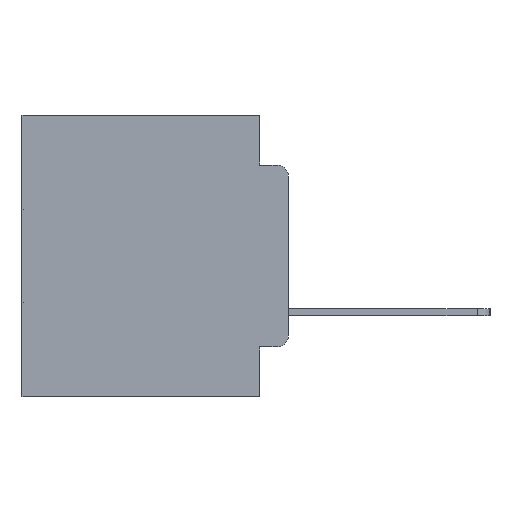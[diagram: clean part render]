
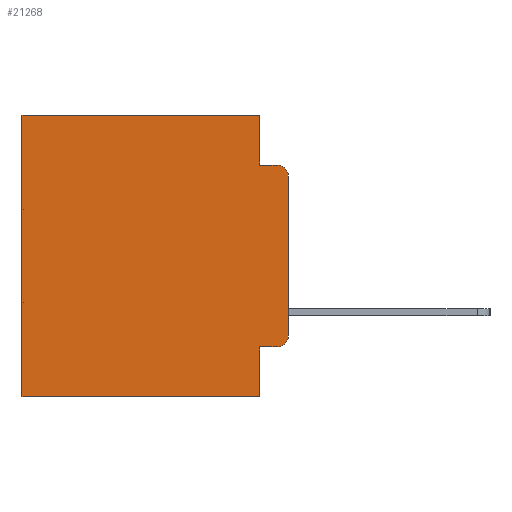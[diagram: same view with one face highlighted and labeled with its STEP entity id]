
A CAD part, left-side view. The second image highlights one B-rep face of the part: STEP entity #21268.
In plain terms, the highlighted planar face has unit normal (-1, 0, 0).
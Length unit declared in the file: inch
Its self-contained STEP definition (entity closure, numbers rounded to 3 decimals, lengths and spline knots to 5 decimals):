
#149 = VECTOR ( 'NONE', #6387, 39.37008 ) ;
#411 = ORIENTED_EDGE ( 'NONE', *, *, #12343, .F. ) ;
#608 = DIRECTION ( 'NONE',  ( 0., 0., -1. ) ) ;
#879 = DIRECTION ( 'NONE',  ( -1., 0., 0. ) ) ;
#1126 = AXIS2_PLACEMENT_3D ( 'NONE', #17650, #3889, #19891 ) ;
#2723 = VERTEX_POINT ( 'NONE', #9617 ) ;
#2884 = VECTOR ( 'NONE', #13279, 39.37008 ) ;
#2995 = ORIENTED_EDGE ( 'NONE', *, *, #27197, .T. ) ;
#3358 = EDGE_CURVE ( 'NONE', #24466, #16225, #23388, .T. ) ;
#3889 = DIRECTION ( 'NONE',  ( -1., 0., 0. ) ) ;
#4315 = VECTOR ( 'NONE', #608, 39.37008 ) ;
#4321 = EDGE_CURVE ( 'NONE', #2723, #8296, #20871, .T. ) ;
#4441 = ORIENTED_EDGE ( 'NONE', *, *, #24781, .F. ) ;
#5885 = ORIENTED_EDGE ( 'NONE', *, *, #16592, .T. ) ;
#5992 = LINE ( 'NONE', #10211, #21342 ) ;
#6387 = DIRECTION ( 'NONE',  ( 0., -1., 0. ) ) ;
#6478 = CARTESIAN_POINT ( 'NONE',  ( 0.298, 0.473, 0. ) ) ;
#6500 = VERTEX_POINT ( 'NONE', #8857 ) ;
#6699 = CARTESIAN_POINT ( 'NONE',  ( 0.298, 0., 0. ) ) ;
#7358 = VERTEX_POINT ( 'NONE', #14186 ) ;
#7810 = AXIS2_PLACEMENT_3D ( 'NONE', #22222, #10803, #13249 ) ;
#8296 = VERTEX_POINT ( 'NONE', #20118 ) ;
#8422 = VERTEX_POINT ( 'NONE', #9274 ) ;
#8857 = CARTESIAN_POINT ( 'NONE',  ( 0.298, 0.051, -0.4115 ) ) ;
#8985 = CARTESIAN_POINT ( 'NONE',  ( 0.298, 0., -0.1085 ) ) ;
#9028 = LINE ( 'NONE', #24500, #2884 ) ;
#9274 = CARTESIAN_POINT ( 'NONE',  ( 0.298, 0.051, -0.5 ) ) ;
#9549 = EDGE_CURVE ( 'NONE', #6500, #24466, #19239, .T. ) ;
#9617 = CARTESIAN_POINT ( 'NONE',  ( 0.298, 0.051, -0.0885 ) ) ;
#9822 = CARTESIAN_POINT ( 'NONE',  ( 0.298, 0.051, 0. ) ) ;
#9849 = ORIENTED_EDGE ( 'NONE', *, *, #4321, .F. ) ;
#10211 = CARTESIAN_POINT ( 'NONE',  ( 0.298, 0., 0. ) ) ;
#10475 = LINE ( 'NONE', #9822, #4315 ) ;
#10803 = DIRECTION ( 'NONE',  ( 1., 0., 0. ) ) ;
#10911 = PLANE ( 'NONE',  #7810 ) ;
#11896 = LINE ( 'NONE', #19379, #17164 ) ;
#12021 = CARTESIAN_POINT ( 'NONE',  ( 0.298, 0.473, 0. ) ) ;
#12343 = EDGE_CURVE ( 'NONE', #8422, #7358, #9028, .T. ) ;
#13090 = VERTEX_POINT ( 'NONE', #6478 ) ;
#13249 = DIRECTION ( 'NONE',  ( 0., 0., -1. ) ) ;
#13279 = DIRECTION ( 'NONE',  ( 0., 1., 0. ) ) ;
#13618 = DIRECTION ( 'NONE',  ( 0., -1., 0. ) ) ;
#14186 = CARTESIAN_POINT ( 'NONE',  ( 0.298, 0.473, -0.5 ) ) ;
#14570 = ORIENTED_EDGE ( 'NONE', *, *, #16103, .F. ) ;
#14743 = CARTESIAN_POINT ( 'NONE',  ( 0.298, 0.02, -0.3915 ) ) ;
#14925 = VECTOR ( 'NONE', #13618, 39.37008 ) ;
#15715 = EDGE_CURVE ( 'NONE', #6500, #8422, #11896, .T. ) ;
#16103 = EDGE_CURVE ( 'NONE', #23313, #16225, #16105, .T. ) ;
#16105 = LINE ( 'NONE', #6699, #20649 ) ;
#16225 = VERTEX_POINT ( 'NONE', #20453 ) ;
#16592 = EDGE_CURVE ( 'NONE', #26869, #13090, #5992, .T. ) ;
#16981 = DIRECTION ( 'NONE',  ( 0., 0., -1. ) ) ;
#17123 = DIRECTION ( 'NONE',  ( 0., 0., -1. ) ) ;
#17164 = VECTOR ( 'NONE', #17123, 39.37008 ) ;
#17650 = CARTESIAN_POINT ( 'NONE',  ( 0.298, 0.02, -0.1085 ) ) ;
#18629 = AXIS2_PLACEMENT_3D ( 'NONE', #14743, #879, #16981 ) ;
#18832 = FACE_OUTER_BOUND ( 'NONE', #26794, .T. ) ;
#19239 = LINE ( 'NONE', #20051, #149 ) ;
#19260 = DIRECTION ( 'NONE',  ( 0., 1., 0. ) ) ;
#19379 = CARTESIAN_POINT ( 'NONE',  ( 0.298, 0.051, 0. ) ) ;
#19891 = DIRECTION ( 'NONE',  ( 0., 0., -1. ) ) ;
#20051 = CARTESIAN_POINT ( 'NONE',  ( 0.298, 0.051, -0.4115 ) ) ;
#20118 = CARTESIAN_POINT ( 'NONE',  ( 0.298, 0.02, -0.0885 ) ) ;
#20185 = ORIENTED_EDGE ( 'NONE', *, *, #15715, .F. ) ;
#20218 = EDGE_CURVE ( 'NONE', #13090, #7358, #22135, .T. ) ;
#20269 = CARTESIAN_POINT ( 'NONE',  ( 0.298, 0.051, -0.0885 ) ) ;
#20453 = CARTESIAN_POINT ( 'NONE',  ( 0.298, 0., -0.3915 ) ) ;
#20495 = CARTESIAN_POINT ( 'NONE',  ( 0.298, 0.051, 0. ) ) ;
#20649 = VECTOR ( 'NONE', #24913, 39.37008 ) ;
#20658 = VECTOR ( 'NONE', #23234, 39.37008 ) ;
#20871 = LINE ( 'NONE', #20269, #14925 ) ;
#21268 = ADVANCED_FACE ( 'NONE', ( #18832 ), #10911, .F. ) ;
#21342 = VECTOR ( 'NONE', #19260, 39.37008 ) ;
#22135 = LINE ( 'NONE', #12021, #20658 ) ;
#22222 = CARTESIAN_POINT ( 'NONE',  ( 0.298, 0., 0. ) ) ;
#22349 = ORIENTED_EDGE ( 'NONE', *, *, #9549, .T. ) ;
#23234 = DIRECTION ( 'NONE',  ( 0., 0., -1. ) ) ;
#23313 = VERTEX_POINT ( 'NONE', #8985 ) ;
#23388 = CIRCLE ( 'NONE', #18629, 0.02 ) ;
#24098 = ORIENTED_EDGE ( 'NONE', *, *, #20218, .T. ) ;
#24466 = VERTEX_POINT ( 'NONE', #26878 ) ;
#24500 = CARTESIAN_POINT ( 'NONE',  ( 0.298, 0., -0.5 ) ) ;
#24781 = EDGE_CURVE ( 'NONE', #26869, #2723, #10475, .T. ) ;
#24913 = DIRECTION ( 'NONE',  ( 0., 0., -1. ) ) ;
#26794 = EDGE_LOOP ( 'NONE', ( #14570, #2995, #9849, #4441, #5885, #24098, #411, #20185, #22349, #28284 ) ) ;
#26869 = VERTEX_POINT ( 'NONE', #20495 ) ;
#26878 = CARTESIAN_POINT ( 'NONE',  ( 0.298, 0.02, -0.4115 ) ) ;
#27197 = EDGE_CURVE ( 'NONE', #23313, #8296, #29393, .T. ) ;
#28284 = ORIENTED_EDGE ( 'NONE', *, *, #3358, .T. ) ;
#29393 = CIRCLE ( 'NONE', #1126, 0.02 ) ;
